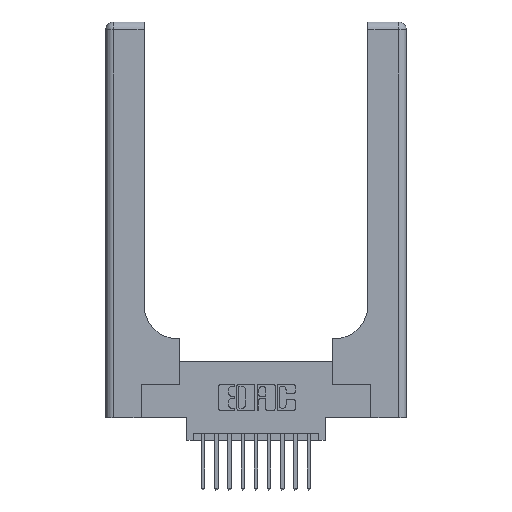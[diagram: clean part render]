
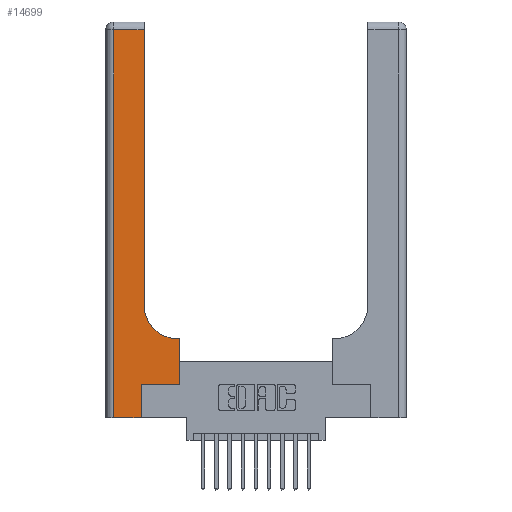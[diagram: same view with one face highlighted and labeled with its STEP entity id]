
A CAD part, top view. The second image highlights one B-rep face of the part: STEP entity #14699.
In plain terms, the highlighted planar face has unit normal (0, 0, 1).
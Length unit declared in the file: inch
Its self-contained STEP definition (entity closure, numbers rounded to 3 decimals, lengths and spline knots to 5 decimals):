
#197 = DIRECTION ( 'NONE',  ( 1., 0., 0. ) ) ;
#459 = ORIENTED_EDGE ( 'NONE', *, *, #3757, .T. ) ;
#568 = VECTOR ( 'NONE', #2304, 39.37008 ) ;
#582 = VECTOR ( 'NONE', #10611, 39.37008 ) ;
#596 = CIRCLE ( 'NONE', #1994, 0.25 ) ;
#886 = CARTESIAN_POINT ( 'NONE',  ( 0.06, 3., 0.37 ) ) ;
#935 = EDGE_LOOP ( 'NONE', ( #3009, #459, #14379, #16706, #1626, #14406, #10197, #2924, #2014 ) ) ;
#1000 = CARTESIAN_POINT ( 'NONE',  ( 0.5585, 0.25, 0.37 ) ) ;
#1311 = LINE ( 'NONE', #2100, #8177 ) ;
#1626 = ORIENTED_EDGE ( 'NONE', *, *, #10285, .T. ) ;
#1825 = VERTEX_POINT ( 'NONE', #9072 ) ;
#1935 = LINE ( 'NONE', #11998, #15341 ) ;
#1994 = AXIS2_PLACEMENT_3D ( 'NONE', #2948, #12175, #4337 ) ;
#2014 = ORIENTED_EDGE ( 'NONE', *, *, #9814, .T. ) ;
#2100 = CARTESIAN_POINT ( 'NONE',  ( 0.2915, 3., 0.37 ) ) ;
#2304 = DIRECTION ( 'NONE',  ( 0., -1., 0. ) ) ;
#2562 = LINE ( 'NONE', #13276, #5818 ) ;
#2744 = DIRECTION ( 'NONE',  ( -1., 0., 0. ) ) ;
#2924 = ORIENTED_EDGE ( 'NONE', *, *, #16172, .T. ) ;
#2948 = CARTESIAN_POINT ( 'NONE',  ( 0.5415, 0.85, 0.37 ) ) ;
#3009 = ORIENTED_EDGE ( 'NONE', *, *, #15125, .T. ) ;
#3757 = EDGE_CURVE ( 'NONE', #8111, #9592, #2562, .T. ) ;
#3957 = CARTESIAN_POINT ( 'NONE',  ( 0.269, 0., 0.37 ) ) ;
#4337 = DIRECTION ( 'NONE',  ( 1., 0., 0. ) ) ;
#4558 = LINE ( 'NONE', #5787, #14413 ) ;
#5137 = CARTESIAN_POINT ( 'NONE',  ( 0.5585, 0.25, 0.37 ) ) ;
#5787 = CARTESIAN_POINT ( 'NONE',  ( 0., 0., 0.37 ) ) ;
#5818 = VECTOR ( 'NONE', #9552, 39.37008 ) ;
#6387 = VERTEX_POINT ( 'NONE', #5137 ) ;
#7440 = VERTEX_POINT ( 'NONE', #14950 ) ;
#7638 = VERTEX_POINT ( 'NONE', #9101 ) ;
#7913 = LINE ( 'NONE', #3957, #582 ) ;
#7924 = CARTESIAN_POINT ( 'NONE',  ( 0., 3., 0.37 ) ) ;
#8111 = VERTEX_POINT ( 'NONE', #16751 ) ;
#8177 = VECTOR ( 'NONE', #12665, 39.37008 ) ;
#8297 = EDGE_CURVE ( 'NONE', #7638, #6387, #11977, .T. ) ;
#8610 = VECTOR ( 'NONE', #197, 39.37008 ) ;
#9042 = CARTESIAN_POINT ( 'NONE',  ( 0.06, 2.94, 0.37 ) ) ;
#9072 = CARTESIAN_POINT ( 'NONE',  ( 0.5415, 0.6, 0.37 ) ) ;
#9101 = CARTESIAN_POINT ( 'NONE',  ( 0.269, 0.25, 0.37 ) ) ;
#9214 = DIRECTION ( 'NONE',  ( -1., 0., 0. ) ) ;
#9552 = DIRECTION ( 'NONE',  ( -1., 0., 0. ) ) ;
#9592 = VERTEX_POINT ( 'NONE', #9042 ) ;
#9696 = EDGE_CURVE ( 'NONE', #6387, #10426, #10132, .T. ) ;
#9753 = VECTOR ( 'NONE', #16753, 39.37008 ) ;
#9814 = EDGE_CURVE ( 'NONE', #1825, #15352, #596, .T. ) ;
#10132 = LINE ( 'NONE', #1000, #9753 ) ;
#10197 = ORIENTED_EDGE ( 'NONE', *, *, #9696, .T. ) ;
#10285 = EDGE_CURVE ( 'NONE', #12100, #7638, #7913, .T. ) ;
#10426 = VERTEX_POINT ( 'NONE', #15886 ) ;
#10611 = DIRECTION ( 'NONE',  ( 0., 1., 0. ) ) ;
#10738 = EDGE_CURVE ( 'NONE', #9592, #7440, #11261, .T. ) ;
#10896 = CARTESIAN_POINT ( 'NONE',  ( 0.269, 0.25, 0.37 ) ) ;
#11145 = FACE_OUTER_BOUND ( 'NONE', #935, .T. ) ;
#11261 = LINE ( 'NONE', #886, #568 ) ;
#11620 = CARTESIAN_POINT ( 'NONE',  ( 0.269, 0., 0.37 ) ) ;
#11852 = CARTESIAN_POINT ( 'NONE',  ( 0.2915, 0.85, 0.37 ) ) ;
#11977 = LINE ( 'NONE', #10896, #8610 ) ;
#11998 = CARTESIAN_POINT ( 'NONE',  ( 0.2915, 0.6, 0.37 ) ) ;
#12100 = VERTEX_POINT ( 'NONE', #11620 ) ;
#12175 = DIRECTION ( 'NONE',  ( 0., 0., -1. ) ) ;
#12665 = DIRECTION ( 'NONE',  ( 0., 1., 0. ) ) ;
#13276 = CARTESIAN_POINT ( 'NONE',  ( 0., 2.94, 0.37 ) ) ;
#13450 = DIRECTION ( 'NONE',  ( 1., 0., 0. ) ) ;
#14379 = ORIENTED_EDGE ( 'NONE', *, *, #10738, .T. ) ;
#14406 = ORIENTED_EDGE ( 'NONE', *, *, #8297, .T. ) ;
#14413 = VECTOR ( 'NONE', #13450, 39.37008 ) ;
#14539 = AXIS2_PLACEMENT_3D ( 'NONE', #7924, #16605, #9214 ) ;
#14699 = ADVANCED_FACE ( 'NONE', ( #11145 ), #15387, .F. ) ;
#14950 = CARTESIAN_POINT ( 'NONE',  ( 0.06, 0., 0.37 ) ) ;
#15125 = EDGE_CURVE ( 'NONE', #15352, #8111, #1311, .T. ) ;
#15341 = VECTOR ( 'NONE', #2744, 39.37008 ) ;
#15352 = VERTEX_POINT ( 'NONE', #11852 ) ;
#15387 = PLANE ( 'NONE',  #14539 ) ;
#15532 = EDGE_CURVE ( 'NONE', #7440, #12100, #4558, .T. ) ;
#15886 = CARTESIAN_POINT ( 'NONE',  ( 0.5585, 0.6, 0.37 ) ) ;
#16172 = EDGE_CURVE ( 'NONE', #10426, #1825, #1935, .T. ) ;
#16605 = DIRECTION ( 'NONE',  ( 0., 0., -1. ) ) ;
#16706 = ORIENTED_EDGE ( 'NONE', *, *, #15532, .T. ) ;
#16751 = CARTESIAN_POINT ( 'NONE',  ( 0.2915, 2.94, 0.37 ) ) ;
#16753 = DIRECTION ( 'NONE',  ( 0., 1., 0. ) ) ;
